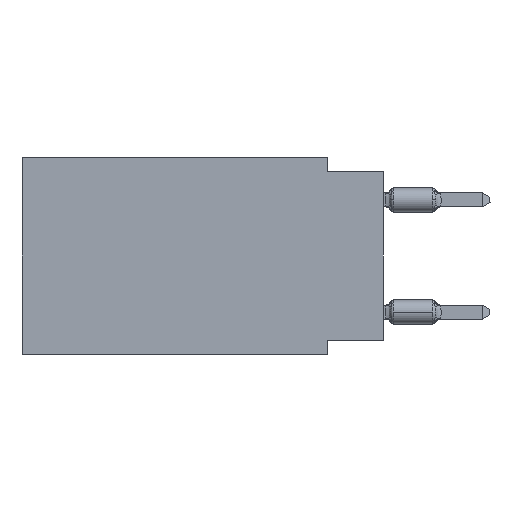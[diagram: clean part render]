
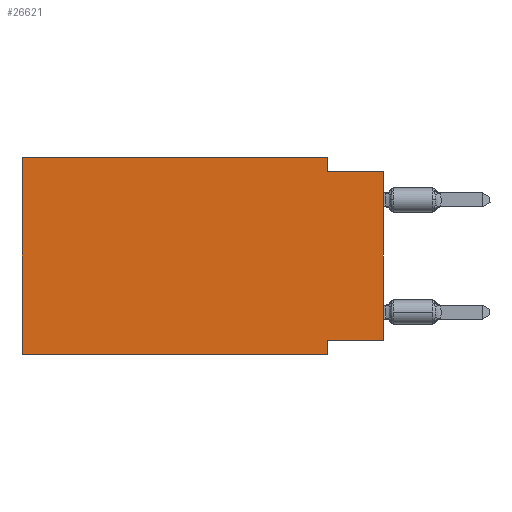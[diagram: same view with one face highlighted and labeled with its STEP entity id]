
A CAD part, left-side view. The second image highlights one B-rep face of the part: STEP entity #26621.
In plain terms, the highlighted planar face has unit normal (-1, 0, 0).
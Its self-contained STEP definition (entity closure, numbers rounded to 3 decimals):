
#31 = VERTEX_POINT ( 'NONE', #11152 ) ;
#1057 = FACE_OUTER_BOUND ( 'NONE', #16949, .T. ) ;
#3512 = VECTOR ( 'NONE', #9575, 1000. ) ;
#4045 = VERTEX_POINT ( 'NONE', #12932 ) ;
#4542 = LINE ( 'NONE', #19548, #20793 ) ;
#6119 = CARTESIAN_POINT ( 'NONE',  ( 0., 16.383, -8.89 ) ) ;
#6265 = VERTEX_POINT ( 'NONE', #31263 ) ;
#6338 = VERTEX_POINT ( 'NONE', #22283 ) ;
#6766 = ORIENTED_EDGE ( 'NONE', *, *, #32322, .T. ) ;
#7212 = DIRECTION ( 'NONE',  ( 0., 1., 0. ) ) ;
#7536 = CARTESIAN_POINT ( 'NONE',  ( 0., 0., -8.255 ) ) ;
#8444 = DIRECTION ( 'NONE',  ( 0., -1., 0. ) ) ;
#8821 = CARTESIAN_POINT ( 'NONE',  ( 0., 16.383, 0. ) ) ;
#9190 = CARTESIAN_POINT ( 'NONE',  ( 0., 2.54, -8.89 ) ) ;
#9329 = VERTEX_POINT ( 'NONE', #8821 ) ;
#9575 = DIRECTION ( 'NONE',  ( 0., -1., 0. ) ) ;
#9869 = DIRECTION ( 'NONE',  ( 0., 0., -1. ) ) ;
#9905 = EDGE_CURVE ( 'NONE', #26662, #6265, #24595, .T. ) ;
#10516 = ORIENTED_EDGE ( 'NONE', *, *, #19299, .T. ) ;
#11152 = CARTESIAN_POINT ( 'NONE',  ( 0., 2.54, -8.89 ) ) ;
#11859 = VECTOR ( 'NONE', #25915, 1000. ) ;
#12433 = CARTESIAN_POINT ( 'NONE',  ( 0., 0., -0.635 ) ) ;
#12932 = CARTESIAN_POINT ( 'NONE',  ( 0., 2.54, -8.255 ) ) ;
#12960 = LINE ( 'NONE', #6119, #13133 ) ;
#13133 = VECTOR ( 'NONE', #8444, 1000. ) ;
#13323 = EDGE_CURVE ( 'NONE', #6338, #9329, #13402, .T. ) ;
#13402 = LINE ( 'NONE', #18229, #11859 ) ;
#14573 = LINE ( 'NONE', #32863, #3512 ) ;
#14607 = DIRECTION ( 'NONE',  ( 0., -1., 0. ) ) ;
#14713 = CARTESIAN_POINT ( 'NONE',  ( 0., 0., -8.255 ) ) ;
#15210 = EDGE_CURVE ( 'NONE', #4045, #31, #29663, .T. ) ;
#16891 = PLANE ( 'NONE',  #21179 ) ;
#16949 = EDGE_LOOP ( 'NONE', ( #6766, #27618, #22400, #25128, #21856, #10516, #32070, #24829 ) ) ;
#18229 = CARTESIAN_POINT ( 'NONE',  ( 0., 16.383, 0. ) ) ;
#18642 = VECTOR ( 'NONE', #9869, 1000. ) ;
#18811 = VECTOR ( 'NONE', #14607, 1000. ) ;
#19299 = EDGE_CURVE ( 'NONE', #6338, #31, #12960, .T. ) ;
#19378 = CARTESIAN_POINT ( 'NONE',  ( 0., 16.383, 0. ) ) ;
#19548 = CARTESIAN_POINT ( 'NONE',  ( 0., 2.54, 0. ) ) ;
#20793 = VECTOR ( 'NONE', #27702, 1000. ) ;
#21179 = AXIS2_PLACEMENT_3D ( 'NONE', #19378, #29036, #21381 ) ;
#21269 = CARTESIAN_POINT ( 'NONE',  ( 0., 0., 0. ) ) ;
#21381 = DIRECTION ( 'NONE',  ( 0., 0., -1. ) ) ;
#21710 = CARTESIAN_POINT ( 'NONE',  ( 0., 2.54, -0.635 ) ) ;
#21856 = ORIENTED_EDGE ( 'NONE', *, *, #13323, .F. ) ;
#22283 = CARTESIAN_POINT ( 'NONE',  ( 0., 16.383, -8.89 ) ) ;
#22290 = VECTOR ( 'NONE', #24087, 1000. ) ;
#22400 = ORIENTED_EDGE ( 'NONE', *, *, #31179, .F. ) ;
#23856 = VECTOR ( 'NONE', #7212, 1000. ) ;
#24087 = DIRECTION ( 'NONE',  ( 0., 0., 1. ) ) ;
#24536 = EDGE_CURVE ( 'NONE', #9329, #26835, #14573, .T. ) ;
#24595 = LINE ( 'NONE', #12433, #18811 ) ;
#24829 = ORIENTED_EDGE ( 'NONE', *, *, #26801, .F. ) ;
#24876 = CARTESIAN_POINT ( 'NONE',  ( 0., 2.54, 0. ) ) ;
#25128 = ORIENTED_EDGE ( 'NONE', *, *, #24536, .F. ) ;
#25915 = DIRECTION ( 'NONE',  ( 0., 0., 1. ) ) ;
#26621 = ADVANCED_FACE ( 'NONE', ( #1057 ), #16891, .F. ) ;
#26662 = VERTEX_POINT ( 'NONE', #21710 ) ;
#26801 = EDGE_CURVE ( 'NONE', #31249, #4045, #32329, .T. ) ;
#26835 = VERTEX_POINT ( 'NONE', #24876 ) ;
#27618 = ORIENTED_EDGE ( 'NONE', *, *, #9905, .F. ) ;
#27702 = DIRECTION ( 'NONE',  ( 0., 0., -1. ) ) ;
#29036 = DIRECTION ( 'NONE',  ( 1., 0., 0. ) ) ;
#29663 = LINE ( 'NONE', #9190, #18642 ) ;
#31179 = EDGE_CURVE ( 'NONE', #26835, #26662, #4542, .T. ) ;
#31249 = VERTEX_POINT ( 'NONE', #7536 ) ;
#31263 = CARTESIAN_POINT ( 'NONE',  ( 0., 0., -0.635 ) ) ;
#31557 = LINE ( 'NONE', #21269, #22290 ) ;
#32070 = ORIENTED_EDGE ( 'NONE', *, *, #15210, .F. ) ;
#32322 = EDGE_CURVE ( 'NONE', #31249, #6265, #31557, .T. ) ;
#32329 = LINE ( 'NONE', #14713, #23856 ) ;
#32863 = CARTESIAN_POINT ( 'NONE',  ( 0., 16.383, 0. ) ) ;
